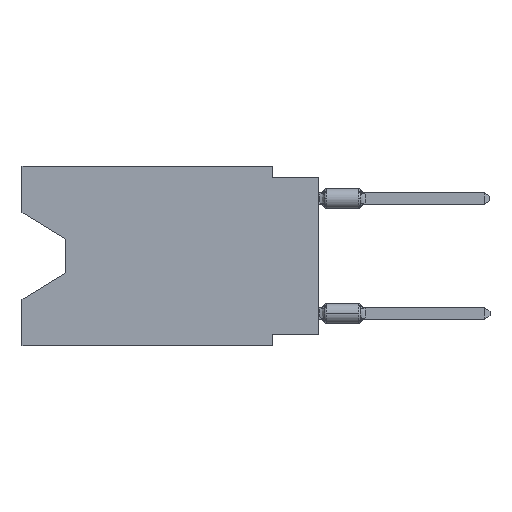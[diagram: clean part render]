
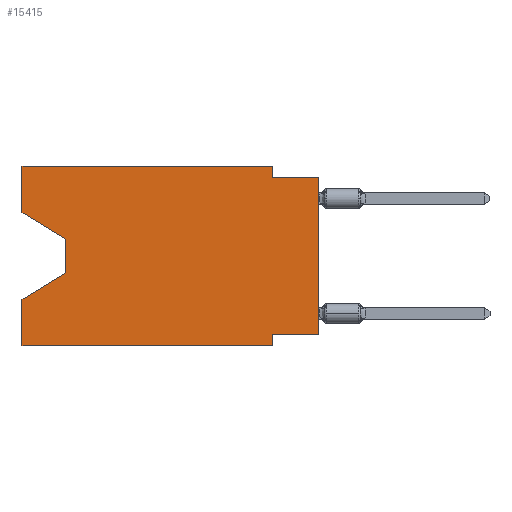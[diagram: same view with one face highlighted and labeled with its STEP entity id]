
A CAD part, left-side view. The second image highlights one B-rep face of the part: STEP entity #15415.
In plain terms, the highlighted planar face has unit normal (-1, 0, 0).
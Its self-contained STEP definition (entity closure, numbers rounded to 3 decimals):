
#54 = VERTEX_POINT ( 'NONE', #422 ) ;
#132 = EDGE_CURVE ( 'NONE', #10444, #54, #7654, .T. ) ;
#317 = CARTESIAN_POINT ( 'NONE',  ( 0., 16.383, 0. ) ) ;
#352 = CARTESIAN_POINT ( 'NONE',  ( 0., 0., -0.635 ) ) ;
#422 = CARTESIAN_POINT ( 'NONE',  ( 0., 2.54, -9.271 ) ) ;
#473 = VECTOR ( 'NONE', #7976, 1000. ) ;
#534 = DIRECTION ( 'NONE',  ( 0., -1., 0. ) ) ;
#567 = VERTEX_POINT ( 'NONE', #13288 ) ;
#813 = VERTEX_POINT ( 'NONE', #1319 ) ;
#892 = CARTESIAN_POINT ( 'NONE',  ( 0., 16.383, 0. ) ) ;
#1077 = VECTOR ( 'NONE', #17481, 1000. ) ;
#1189 = VECTOR ( 'NONE', #534, 1000. ) ;
#1319 = CARTESIAN_POINT ( 'NONE',  ( 0., 16.383, -7.36 ) ) ;
#1862 = EDGE_CURVE ( 'NONE', #11381, #813, #4896, .T. ) ;
#2005 = DIRECTION ( 'NONE',  ( 0., 0., -1. ) ) ;
#2053 = CARTESIAN_POINT ( 'NONE',  ( 0., 16.383, -9.906 ) ) ;
#2126 = LINE ( 'NONE', #352, #1189 ) ;
#2804 = LINE ( 'NONE', #10335, #10554 ) ;
#2964 = CARTESIAN_POINT ( 'NONE',  ( 0., 16.383, -2.546 ) ) ;
#3622 = EDGE_CURVE ( 'NONE', #567, #16390, #14942, .T. ) ;
#3775 = EDGE_CURVE ( 'NONE', #54, #16390, #12230, .T. ) ;
#3922 = DIRECTION ( 'NONE',  ( 0., 0., -1. ) ) ;
#3929 = VECTOR ( 'NONE', #3922, 1000. ) ;
#4328 = CARTESIAN_POINT ( 'NONE',  ( 0., 16.383, 0. ) ) ;
#4590 = DIRECTION ( 'NONE',  ( 0., 0., -1. ) ) ;
#4896 = LINE ( 'NONE', #16286, #5821 ) ;
#5251 = CARTESIAN_POINT ( 'NONE',  ( 0., 2.54, -9.906 ) ) ;
#5821 = VECTOR ( 'NONE', #6036, 1000. ) ;
#5941 = LINE ( 'NONE', #16287, #12284 ) ;
#6007 = LINE ( 'NONE', #17474, #12958 ) ;
#6036 = DIRECTION ( 'NONE',  ( 0., 0.855, -0.519 ) ) ;
#6424 = CARTESIAN_POINT ( 'NONE',  ( 0., 16.383, 0. ) ) ;
#7232 = CARTESIAN_POINT ( 'NONE',  ( 0., 13.97, -5.893 ) ) ;
#7561 = PLANE ( 'NONE',  #16529 ) ;
#7654 = LINE ( 'NONE', #10671, #8182 ) ;
#7976 = DIRECTION ( 'NONE',  ( 0., 0., -1. ) ) ;
#8061 = ORIENTED_EDGE ( 'NONE', *, *, #3775, .F. ) ;
#8062 = VERTEX_POINT ( 'NONE', #16235 ) ;
#8182 = VECTOR ( 'NONE', #14996, 1000. ) ;
#8717 = DIRECTION ( 'NONE',  ( 0., -0.855, -0.519 ) ) ;
#9076 = VERTEX_POINT ( 'NONE', #11207 ) ;
#9329 = CARTESIAN_POINT ( 'NONE',  ( 0., 13.97, -4.013 ) ) ;
#9797 = VECTOR ( 'NONE', #8717, 1000. ) ;
#10300 = FACE_OUTER_BOUND ( 'NONE', #11224, .T. ) ;
#10335 = CARTESIAN_POINT ( 'NONE',  ( 0., 16.383, 0. ) ) ;
#10444 = VERTEX_POINT ( 'NONE', #13165 ) ;
#10554 = VECTOR ( 'NONE', #18518, 1000. ) ;
#10671 = CARTESIAN_POINT ( 'NONE',  ( 0., 0., -9.271 ) ) ;
#11149 = DIRECTION ( 'NONE',  ( 0., 0., 1. ) ) ;
#11207 = CARTESIAN_POINT ( 'NONE',  ( 0., 2.54, -0.635 ) ) ;
#11224 = EDGE_LOOP ( 'NONE', ( #12862, #11244, #15027, #13239, #15557, #8061, #13424, #17281, #13615, #16233, #13564, #15069 ) ) ;
#11244 = ORIENTED_EDGE ( 'NONE', *, *, #11432, .T. ) ;
#11368 = EDGE_CURVE ( 'NONE', #17104, #17108, #2804, .T. ) ;
#11381 = VERTEX_POINT ( 'NONE', #7232 ) ;
#11432 = EDGE_CURVE ( 'NONE', #12312, #11381, #6007, .T. ) ;
#11915 = VECTOR ( 'NONE', #12909, 1000. ) ;
#12230 = LINE ( 'NONE', #5251, #473 ) ;
#12284 = VECTOR ( 'NONE', #16010, 1000. ) ;
#12312 = VERTEX_POINT ( 'NONE', #9329 ) ;
#12467 = LINE ( 'NONE', #892, #15464 ) ;
#12489 = LINE ( 'NONE', #15194, #3929 ) ;
#12862 = ORIENTED_EDGE ( 'NONE', *, *, #17789, .T. ) ;
#12909 = DIRECTION ( 'NONE',  ( 0., 0., 1. ) ) ;
#12958 = VECTOR ( 'NONE', #4590, 1000. ) ;
#12965 = CARTESIAN_POINT ( 'NONE',  ( 0., 0., -0.635 ) ) ;
#13165 = CARTESIAN_POINT ( 'NONE',  ( 0., 0., -9.271 ) ) ;
#13239 = ORIENTED_EDGE ( 'NONE', *, *, #18408, .F. ) ;
#13288 = CARTESIAN_POINT ( 'NONE',  ( 0., 16.383, -9.906 ) ) ;
#13424 = ORIENTED_EDGE ( 'NONE', *, *, #132, .F. ) ;
#13564 = ORIENTED_EDGE ( 'NONE', *, *, #11368, .F. ) ;
#13615 = ORIENTED_EDGE ( 'NONE', *, *, #14974, .F. ) ;
#13783 = EDGE_CURVE ( 'NONE', #10444, #14835, #5941, .T. ) ;
#14802 = DIRECTION ( 'NONE',  ( 1., 0., 0. ) ) ;
#14835 = VERTEX_POINT ( 'NONE', #12965 ) ;
#14942 = LINE ( 'NONE', #2053, #1077 ) ;
#14974 = EDGE_CURVE ( 'NONE', #9076, #14835, #2126, .T. ) ;
#14996 = DIRECTION ( 'NONE',  ( 0., 1., 0. ) ) ;
#15027 = ORIENTED_EDGE ( 'NONE', *, *, #1862, .T. ) ;
#15069 = ORIENTED_EDGE ( 'NONE', *, *, #16808, .F. ) ;
#15194 = CARTESIAN_POINT ( 'NONE',  ( 0., 2.54, 0. ) ) ;
#15415 = ADVANCED_FACE ( 'NONE', ( #10300 ), #7561, .F. ) ;
#15464 = VECTOR ( 'NONE', #11149, 1000. ) ;
#15557 = ORIENTED_EDGE ( 'NONE', *, *, #3622, .T. ) ;
#15861 = LINE ( 'NONE', #2964, #9797 ) ;
#16010 = DIRECTION ( 'NONE',  ( 0., 0., 1. ) ) ;
#16233 = ORIENTED_EDGE ( 'NONE', *, *, #16351, .F. ) ;
#16235 = CARTESIAN_POINT ( 'NONE',  ( 0., 16.383, -2.546 ) ) ;
#16286 = CARTESIAN_POINT ( 'NONE',  ( 0., 13.97, -5.893 ) ) ;
#16287 = CARTESIAN_POINT ( 'NONE',  ( 0., 0., 0. ) ) ;
#16351 = EDGE_CURVE ( 'NONE', #17108, #9076, #12489, .T. ) ;
#16390 = VERTEX_POINT ( 'NONE', #18211 ) ;
#16529 = AXIS2_PLACEMENT_3D ( 'NONE', #6424, #14802, #2005 ) ;
#16760 = LINE ( 'NONE', #4328, #11915 ) ;
#16808 = EDGE_CURVE ( 'NONE', #8062, #17104, #12467, .T. ) ;
#17104 = VERTEX_POINT ( 'NONE', #317 ) ;
#17108 = VERTEX_POINT ( 'NONE', #17603 ) ;
#17281 = ORIENTED_EDGE ( 'NONE', *, *, #13783, .T. ) ;
#17474 = CARTESIAN_POINT ( 'NONE',  ( 0., 13.97, -4.013 ) ) ;
#17481 = DIRECTION ( 'NONE',  ( 0., -1., 0. ) ) ;
#17603 = CARTESIAN_POINT ( 'NONE',  ( 0., 2.54, 0. ) ) ;
#17789 = EDGE_CURVE ( 'NONE', #8062, #12312, #15861, .T. ) ;
#18211 = CARTESIAN_POINT ( 'NONE',  ( 0., 2.54, -9.906 ) ) ;
#18408 = EDGE_CURVE ( 'NONE', #567, #813, #16760, .T. ) ;
#18518 = DIRECTION ( 'NONE',  ( 0., -1., 0. ) ) ;
